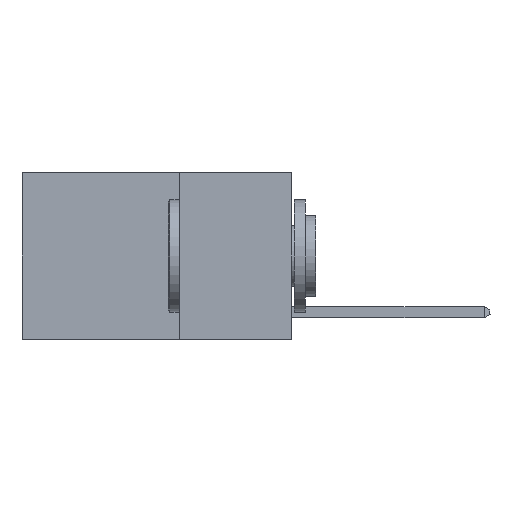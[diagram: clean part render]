
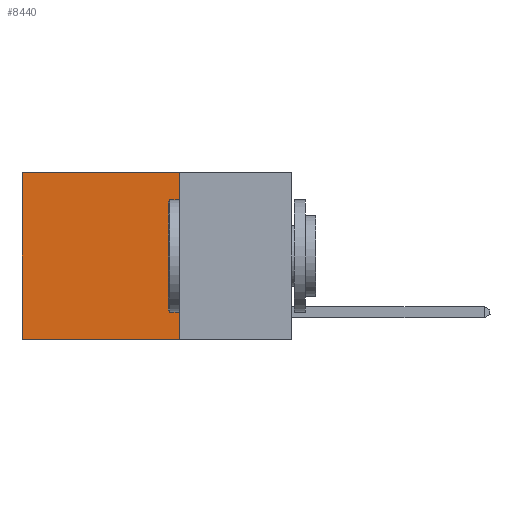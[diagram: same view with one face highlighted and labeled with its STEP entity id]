
A CAD part, left-side view. The second image highlights one B-rep face of the part: STEP entity #8440.
In plain terms, the highlighted planar face has unit normal (-1, 0, 0).
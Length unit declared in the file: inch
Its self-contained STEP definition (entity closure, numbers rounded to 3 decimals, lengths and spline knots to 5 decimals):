
#1667 = CARTESIAN_POINT ( 'NONE',  ( 0.2625, 0.25, -0.37 ) ) ;
#2407 = EDGE_CURVE ( 'NONE', #8634, #5355, #4995, .T. ) ;
#2770 = CARTESIAN_POINT ( 'NONE',  ( 0.2625, 0.25, 0. ) ) ;
#2902 = VECTOR ( 'NONE', #17113, 39.37008 ) ;
#3787 = EDGE_CURVE ( 'NONE', #19403, #5355, #7737, .T. ) ;
#4532 = DIRECTION ( 'NONE',  ( 1., 0., 0. ) ) ;
#4995 = LINE ( 'NONE', #17927, #19130 ) ;
#5355 = VERTEX_POINT ( 'NONE', #19001 ) ;
#6430 = DIRECTION ( 'NONE',  ( 0., 0., -1. ) ) ;
#7737 = LINE ( 'NONE', #11399, #10171 ) ;
#7842 = FACE_OUTER_BOUND ( 'NONE', #19030, .T. ) ;
#8440 = ADVANCED_FACE ( 'NONE', ( #7842 ), #17910, .F. ) ;
#8524 = LINE ( 'NONE', #10177, #19420 ) ;
#8634 = VERTEX_POINT ( 'NONE', #1667 ) ;
#10045 = LINE ( 'NONE', #16786, #2902 ) ;
#10048 = CARTESIAN_POINT ( 'NONE',  ( 0.2625, 0.25, 0. ) ) ;
#10171 = VECTOR ( 'NONE', #6430, 39.37008 ) ;
#10177 = CARTESIAN_POINT ( 'NONE',  ( 0.2625, 0.25, 0. ) ) ;
#11399 = CARTESIAN_POINT ( 'NONE',  ( 0.2625, 0.6, 0. ) ) ;
#11622 = AXIS2_PLACEMENT_3D ( 'NONE', #2770, #4532, #13042 ) ;
#11730 = DIRECTION ( 'NONE',  ( 0., 1., 0. ) ) ;
#11814 = ORIENTED_EDGE ( 'NONE', *, *, #2407, .F. ) ;
#12319 = ORIENTED_EDGE ( 'NONE', *, *, #12709, .F. ) ;
#12709 = EDGE_CURVE ( 'NONE', #13961, #8634, #10045, .T. ) ;
#13042 = DIRECTION ( 'NONE',  ( 0., 0., -1. ) ) ;
#13611 = ORIENTED_EDGE ( 'NONE', *, *, #3787, .T. ) ;
#13826 = DIRECTION ( 'NONE',  ( 0., 1., 0. ) ) ;
#13961 = VERTEX_POINT ( 'NONE', #10048 ) ;
#14750 = ORIENTED_EDGE ( 'NONE', *, *, #17832, .T. ) ;
#16786 = CARTESIAN_POINT ( 'NONE',  ( 0.2625, 0.25, 0. ) ) ;
#17113 = DIRECTION ( 'NONE',  ( 0., 0., -1. ) ) ;
#17585 = CARTESIAN_POINT ( 'NONE',  ( 0.2625, 0.6, 0. ) ) ;
#17832 = EDGE_CURVE ( 'NONE', #13961, #19403, #8524, .T. ) ;
#17910 = PLANE ( 'NONE',  #11622 ) ;
#17927 = CARTESIAN_POINT ( 'NONE',  ( 0.2625, 0.25, -0.37 ) ) ;
#19001 = CARTESIAN_POINT ( 'NONE',  ( 0.2625, 0.6, -0.37 ) ) ;
#19030 = EDGE_LOOP ( 'NONE', ( #13611, #11814, #12319, #14750 ) ) ;
#19130 = VECTOR ( 'NONE', #13826, 39.37008 ) ;
#19403 = VERTEX_POINT ( 'NONE', #17585 ) ;
#19420 = VECTOR ( 'NONE', #11730, 39.37008 ) ;
